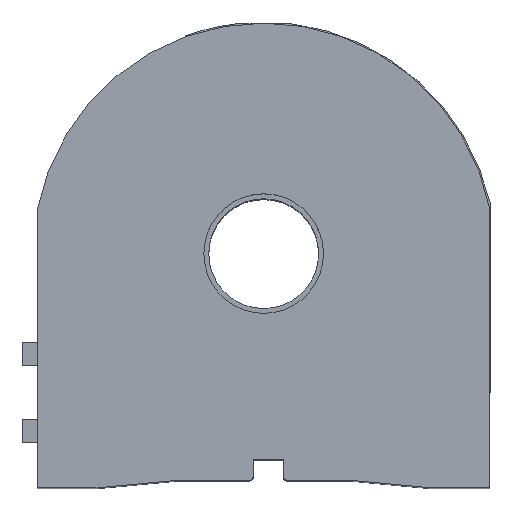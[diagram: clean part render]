
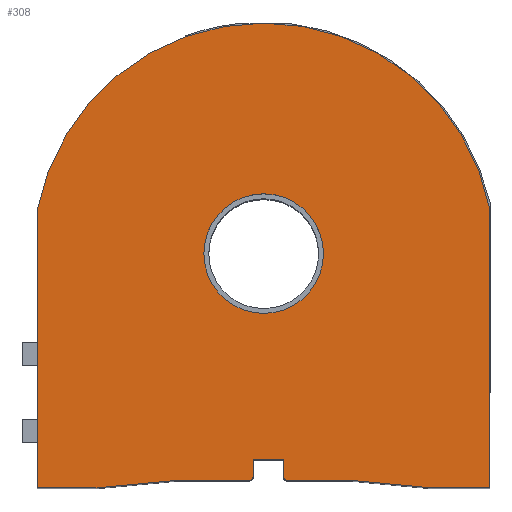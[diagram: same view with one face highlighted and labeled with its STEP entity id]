
A CAD part, top view. The second image highlights one B-rep face of the part: STEP entity #308.
In plain terms, the highlighted planar face has unit normal (0, 0, 1).
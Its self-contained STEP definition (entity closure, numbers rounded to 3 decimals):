
#2 = CARTESIAN_POINT ( 'NONE',  ( -2.75, -53.5, 80. ) ) ;
#40 = ORIENTED_EDGE ( 'NONE', *, *, #288, .T. ) ;
#41 = CIRCLE ( 'NONE', #1725, 15.56 ) ;
#98 = EDGE_CURVE ( 'NONE', #3142, #2666, #3020, .T. ) ;
#116 = ORIENTED_EDGE ( 'NONE', *, *, #2895, .F. ) ;
#121 = LINE ( 'NONE', #682, #1188 ) ;
#147 = CARTESIAN_POINT ( 'NONE',  ( 0., 0., 80. ) ) ;
#163 = ORIENTED_EDGE ( 'NONE', *, *, #1113, .T. ) ;
#188 = LINE ( 'NONE', #3623, #2978 ) ;
#244 = VERTEX_POINT ( 'NONE', #2885 ) ;
#288 = EDGE_CURVE ( 'NONE', #2666, #1952, #1077, .T. ) ;
#307 = DIRECTION ( 'NONE',  ( 0., -1., 0. ) ) ;
#308 = ADVANCED_FACE ( 'NONE', ( #2261, #2861 ), #1987, .F. ) ;
#336 = CARTESIAN_POINT ( 'NONE',  ( -3.75, -58., 80. ) ) ;
#349 = AXIS2_PLACEMENT_3D ( 'NONE', #147, #914, #2051 ) ;
#361 = VERTEX_POINT ( 'NONE', #2 ) ;
#459 = LINE ( 'NONE', #1574, #3518 ) ;
#460 = VECTOR ( 'NONE', #3140, 1000. ) ;
#463 = CARTESIAN_POINT ( 'NONE',  ( 6.083, -58., 80. ) ) ;
#474 = ORIENTED_EDGE ( 'NONE', *, *, #1548, .F. ) ;
#517 = CIRCLE ( 'NONE', #1498, 1. ) ;
#533 = AXIS2_PLACEMENT_3D ( 'NONE', #1694, #2585, #1165 ) ;
#566 = CARTESIAN_POINT ( 'NONE',  ( -2.75, -53.5, 80. ) ) ;
#577 = DIRECTION ( 'NONE',  ( -1., 0., 0. ) ) ;
#601 = DIRECTION ( 'NONE',  ( 0., 0., 1. ) ) ;
#602 = VECTOR ( 'NONE', #611, 1000. ) ;
#611 = DIRECTION ( 'NONE',  ( -0.996, -0.093, 0. ) ) ;
#612 = CARTESIAN_POINT ( 'NONE',  ( 43.909, -61., 80. ) ) ;
#645 = VECTOR ( 'NONE', #1432, 1000. ) ;
#682 = CARTESIAN_POINT ( 'NONE',  ( -58.909, -61., 80. ) ) ;
#705 = VECTOR ( 'NONE', #2262, 1000. ) ;
#766 = CARTESIAN_POINT ( 'NONE',  ( -58.909, -61., 80. ) ) ;
#771 = EDGE_LOOP ( 'NONE', ( #2165, #163, #1943, #1585, #3493, #3252, #40, #3630, #2794, #2837, #1791, #2580, #474, #2942 ) ) ;
#813 = VECTOR ( 'NONE', #307, 1000. ) ;
#836 = AXIS2_PLACEMENT_3D ( 'NONE', #3431, #3111, #577 ) ;
#914 = DIRECTION ( 'NONE',  ( 0., 0., 1. ) ) ;
#970 = DIRECTION ( 'NONE',  ( 0., -1., 0. ) ) ;
#971 = DIRECTION ( 'NONE',  ( 0., 0., 1. ) ) ;
#973 = VERTEX_POINT ( 'NONE', #1220 ) ;
#984 = EDGE_CURVE ( 'NONE', #2855, #3142, #1524, .T. ) ;
#1002 = CARTESIAN_POINT ( 'NONE',  ( -15.56, 0., 80. ) ) ;
#1012 = DIRECTION ( 'NONE',  ( -1., 0., 0. ) ) ;
#1039 = VERTEX_POINT ( 'NONE', #3601 ) ;
#1043 = DIRECTION ( 'NONE',  ( -1., 0., 0. ) ) ;
#1053 = DIRECTION ( 'NONE',  ( -0.996, 0.093, 0. ) ) ;
#1069 = ORIENTED_EDGE ( 'NONE', *, *, #3700, .F. ) ;
#1077 = CIRCLE ( 'NONE', #836, 60. ) ;
#1083 = VECTOR ( 'NONE', #1539, 1000. ) ;
#1113 = EDGE_CURVE ( 'NONE', #2898, #1039, #1921, .T. ) ;
#1128 = CARTESIAN_POINT ( 'NONE',  ( 22.5, -59., 80. ) ) ;
#1165 = DIRECTION ( 'NONE',  ( -1., 0., 0. ) ) ;
#1170 = EDGE_LOOP ( 'NONE', ( #1069, #116 ) ) ;
#1188 = VECTOR ( 'NONE', #970, 1000. ) ;
#1212 = EDGE_CURVE ( 'NONE', #1282, #244, #2064, .T. ) ;
#1220 = CARTESIAN_POINT ( 'NONE',  ( 22.5, -59., 80. ) ) ;
#1272 = CARTESIAN_POINT ( 'NONE',  ( -2.75, -58., 80. ) ) ;
#1282 = VERTEX_POINT ( 'NONE', #3230 ) ;
#1317 = VERTEX_POINT ( 'NONE', #1002 ) ;
#1358 = CARTESIAN_POINT ( 'NONE',  ( 5.083, -66.165, 80. ) ) ;
#1368 = CARTESIAN_POINT ( 'NONE',  ( 58.909, 11.39, 80. ) ) ;
#1432 = DIRECTION ( 'NONE',  ( -1., 0., 0. ) ) ;
#1476 = LINE ( 'NONE', #566, #813 ) ;
#1498 = AXIS2_PLACEMENT_3D ( 'NONE', #336, #601, #3413 ) ;
#1524 = LINE ( 'NONE', #2899, #1083 ) ;
#1539 = DIRECTION ( 'NONE',  ( 1., 0., 0. ) ) ;
#1548 = EDGE_CURVE ( 'NONE', #361, #2480, #1476, .T. ) ;
#1574 = CARTESIAN_POINT ( 'NONE',  ( 5.083, -53.5, 80. ) ) ;
#1585 = ORIENTED_EDGE ( 'NONE', *, *, #1955, .F. ) ;
#1686 = CARTESIAN_POINT ( 'NONE',  ( 15.56, 0., 80. ) ) ;
#1694 = CARTESIAN_POINT ( 'NONE',  ( 0., 0., 80. ) ) ;
#1725 = AXIS2_PLACEMENT_3D ( 'NONE', #3540, #971, #3195 ) ;
#1767 = LINE ( 'NONE', #2057, #645 ) ;
#1791 = ORIENTED_EDGE ( 'NONE', *, *, #3189, .F. ) ;
#1921 = CIRCLE ( 'NONE', #3598, 1. ) ;
#1943 = ORIENTED_EDGE ( 'NONE', *, *, #3262, .F. ) ;
#1948 = DIRECTION ( 'NONE',  ( 0., 1., 0. ) ) ;
#1952 = VERTEX_POINT ( 'NONE', #2756 ) ;
#1955 = EDGE_CURVE ( 'NONE', #2855, #973, #188, .T. ) ;
#1962 = CIRCLE ( 'NONE', #349, 15.56 ) ;
#1987 = PLANE ( 'NONE',  #533 ) ;
#2051 = DIRECTION ( 'NONE',  ( 1., 0., 0. ) ) ;
#2057 = CARTESIAN_POINT ( 'NONE',  ( 22.5, -59., 80. ) ) ;
#2064 = LINE ( 'NONE', #3439, #602 ) ;
#2144 = VECTOR ( 'NONE', #1948, 1000. ) ;
#2165 = ORIENTED_EDGE ( 'NONE', *, *, #3077, .F. ) ;
#2198 = VECTOR ( 'NONE', #3359, 1000. ) ;
#2261 = FACE_BOUND ( 'NONE', #1170, .T. ) ;
#2262 = DIRECTION ( 'NONE',  ( -1., 0., 0. ) ) ;
#2279 = VERTEX_POINT ( 'NONE', #766 ) ;
#2284 = VERTEX_POINT ( 'NONE', #3368 ) ;
#2343 = LINE ( 'NONE', #1128, #705 ) ;
#2466 = CARTESIAN_POINT ( 'NONE',  ( -3.75, -59., 80. ) ) ;
#2479 = EDGE_CURVE ( 'NONE', #1952, #2279, #121, .T. ) ;
#2480 = VERTEX_POINT ( 'NONE', #1272 ) ;
#2560 = VERTEX_POINT ( 'NONE', #2466 ) ;
#2580 = ORIENTED_EDGE ( 'NONE', *, *, #3190, .T. ) ;
#2585 = DIRECTION ( 'NONE',  ( 0., 0., -1. ) ) ;
#2594 = EDGE_CURVE ( 'NONE', #2284, #361, #459, .T. ) ;
#2600 = LINE ( 'NONE', #3387, #460 ) ;
#2666 = VERTEX_POINT ( 'NONE', #1368 ) ;
#2736 = LINE ( 'NONE', #1358, #2198 ) ;
#2756 = CARTESIAN_POINT ( 'NONE',  ( -58.909, 11.39, 80. ) ) ;
#2794 = ORIENTED_EDGE ( 'NONE', *, *, #3507, .T. ) ;
#2807 = VERTEX_POINT ( 'NONE', #1686 ) ;
#2837 = ORIENTED_EDGE ( 'NONE', *, *, #1212, .F. ) ;
#2855 = VERTEX_POINT ( 'NONE', #612 ) ;
#2861 = FACE_OUTER_BOUND ( 'NONE', #771, .T. ) ;
#2885 = CARTESIAN_POINT ( 'NONE',  ( -43.909, -61., 80. ) ) ;
#2895 = EDGE_CURVE ( 'NONE', #1317, #2807, #1962, .T. ) ;
#2898 = VERTEX_POINT ( 'NONE', #3007 ) ;
#2899 = CARTESIAN_POINT ( 'NONE',  ( 58.909, -61., 80. ) ) ;
#2942 = ORIENTED_EDGE ( 'NONE', *, *, #2594, .F. ) ;
#2978 = VECTOR ( 'NONE', #1053, 1000. ) ;
#3007 = CARTESIAN_POINT ( 'NONE',  ( 5.083, -58., 80. ) ) ;
#3020 = LINE ( 'NONE', #3058, #2144 ) ;
#3042 = CARTESIAN_POINT ( 'NONE',  ( 58.909, -61., 80. ) ) ;
#3058 = CARTESIAN_POINT ( 'NONE',  ( 58.909, -61., 80. ) ) ;
#3077 = EDGE_CURVE ( 'NONE', #2898, #2284, #2736, .T. ) ;
#3111 = DIRECTION ( 'NONE',  ( 0., 0., 1. ) ) ;
#3140 = DIRECTION ( 'NONE',  ( 1., 0., 0. ) ) ;
#3142 = VERTEX_POINT ( 'NONE', #3042 ) ;
#3189 = EDGE_CURVE ( 'NONE', #2560, #1282, #1767, .T. ) ;
#3190 = EDGE_CURVE ( 'NONE', #2560, #2480, #517, .T. ) ;
#3195 = DIRECTION ( 'NONE',  ( 1., 0., 0. ) ) ;
#3230 = CARTESIAN_POINT ( 'NONE',  ( -22.5, -59., 80. ) ) ;
#3252 = ORIENTED_EDGE ( 'NONE', *, *, #98, .T. ) ;
#3262 = EDGE_CURVE ( 'NONE', #973, #1039, #2343, .T. ) ;
#3359 = DIRECTION ( 'NONE',  ( 0., 1., 0. ) ) ;
#3368 = CARTESIAN_POINT ( 'NONE',  ( 5.083, -53.5, 80. ) ) ;
#3387 = CARTESIAN_POINT ( 'NONE',  ( 58.909, -61., 80. ) ) ;
#3413 = DIRECTION ( 'NONE',  ( -1., 0., 0. ) ) ;
#3431 = CARTESIAN_POINT ( 'NONE',  ( 0., 0., 80. ) ) ;
#3439 = CARTESIAN_POINT ( 'NONE',  ( -43.909, -61., 80. ) ) ;
#3493 = ORIENTED_EDGE ( 'NONE', *, *, #984, .T. ) ;
#3507 = EDGE_CURVE ( 'NONE', #2279, #244, #2600, .T. ) ;
#3518 = VECTOR ( 'NONE', #1043, 1000. ) ;
#3540 = CARTESIAN_POINT ( 'NONE',  ( 0., 0., 80. ) ) ;
#3578 = DIRECTION ( 'NONE',  ( 0., 0., 1. ) ) ;
#3598 = AXIS2_PLACEMENT_3D ( 'NONE', #463, #3578, #1012 ) ;
#3601 = CARTESIAN_POINT ( 'NONE',  ( 6.083, -59., 80. ) ) ;
#3623 = CARTESIAN_POINT ( 'NONE',  ( 43.909, -61., 80. ) ) ;
#3630 = ORIENTED_EDGE ( 'NONE', *, *, #2479, .T. ) ;
#3700 = EDGE_CURVE ( 'NONE', #2807, #1317, #41, .T. ) ;
